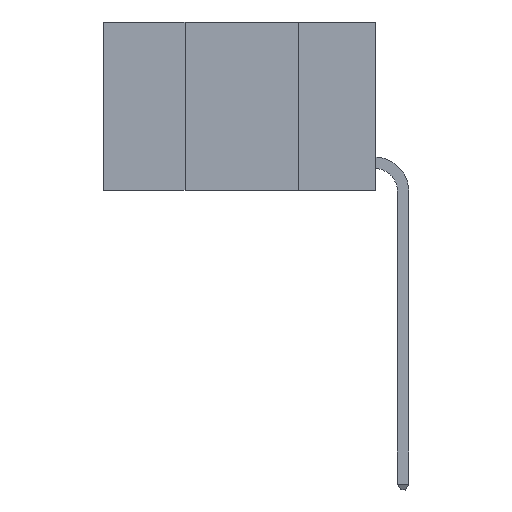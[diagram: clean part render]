
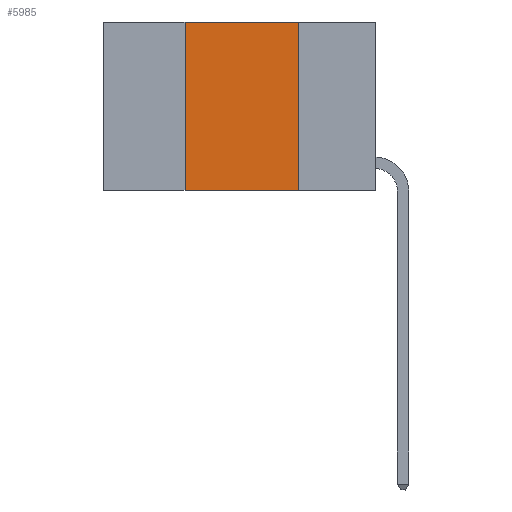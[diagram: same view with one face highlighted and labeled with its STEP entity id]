
A CAD part, left-side view. The second image highlights one B-rep face of the part: STEP entity #5985.
In plain terms, the highlighted planar face has unit normal (-1, 0, 0).
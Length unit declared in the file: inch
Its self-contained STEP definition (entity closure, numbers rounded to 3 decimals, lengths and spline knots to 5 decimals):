
#903 = EDGE_CURVE ( 'NONE', #20603, #3612, #24682, .T. ) ;
#1242 = VECTOR ( 'NONE', #6679, 39.37008 ) ;
#2431 = EDGE_LOOP ( 'NONE', ( #13528, #14172, #3925, #9391 ) ) ;
#2809 = EDGE_CURVE ( 'NONE', #20603, #3908, #10894, .T. ) ;
#2870 = VECTOR ( 'NONE', #26434, 39.37008 ) ;
#3612 = VERTEX_POINT ( 'NONE', #19601 ) ;
#3908 = VERTEX_POINT ( 'NONE', #14766 ) ;
#3925 = ORIENTED_EDGE ( 'NONE', *, *, #903, .F. ) ;
#4415 = LINE ( 'NONE', #21810, #20120 ) ;
#4591 = CARTESIAN_POINT ( 'NONE',  ( 0., 0.6, -0.37 ) ) ;
#5467 = PLANE ( 'NONE',  #12475 ) ;
#5985 = ADVANCED_FACE ( 'NONE', ( #19753 ), #5467, .F. ) ;
#6679 = DIRECTION ( 'NONE',  ( 0., -1., 0. ) ) ;
#7972 = CARTESIAN_POINT ( 'NONE',  ( 0., 0.42, -0.37 ) ) ;
#9391 = ORIENTED_EDGE ( 'NONE', *, *, #2809, .T. ) ;
#9585 = DIRECTION ( 'NONE',  ( 1., 0., 0. ) ) ;
#10894 = LINE ( 'NONE', #4591, #1242 ) ;
#12475 = AXIS2_PLACEMENT_3D ( 'NONE', #25811, #9585, #23859 ) ;
#13189 = VECTOR ( 'NONE', #19718, 39.37008 ) ;
#13528 = ORIENTED_EDGE ( 'NONE', *, *, #16050, .F. ) ;
#14172 = ORIENTED_EDGE ( 'NONE', *, *, #20093, .F. ) ;
#14766 = CARTESIAN_POINT ( 'NONE',  ( 0., 0.17, -0.37 ) ) ;
#16050 = EDGE_CURVE ( 'NONE', #23340, #3908, #24623, .T. ) ;
#16878 = CARTESIAN_POINT ( 'NONE',  ( 0., 0.17, 0. ) ) ;
#17660 = CARTESIAN_POINT ( 'NONE',  ( 0., 0.42, 0. ) ) ;
#19601 = CARTESIAN_POINT ( 'NONE',  ( 0., 0.42, 0. ) ) ;
#19718 = DIRECTION ( 'NONE',  ( 0., 0., 1. ) ) ;
#19753 = FACE_OUTER_BOUND ( 'NONE', #2431, .T. ) ;
#20093 = EDGE_CURVE ( 'NONE', #3612, #23340, #4415, .T. ) ;
#20120 = VECTOR ( 'NONE', #23864, 39.37008 ) ;
#20603 = VERTEX_POINT ( 'NONE', #7972 ) ;
#21810 = CARTESIAN_POINT ( 'NONE',  ( 0., 0.6, 0. ) ) ;
#23340 = VERTEX_POINT ( 'NONE', #16878 ) ;
#23859 = DIRECTION ( 'NONE',  ( 0., 0., -1. ) ) ;
#23864 = DIRECTION ( 'NONE',  ( 0., -1., 0. ) ) ;
#24386 = CARTESIAN_POINT ( 'NONE',  ( 0., 0.17, 0. ) ) ;
#24623 = LINE ( 'NONE', #24386, #2870 ) ;
#24682 = LINE ( 'NONE', #17660, #13189 ) ;
#25811 = CARTESIAN_POINT ( 'NONE',  ( 0., 0.6, 0. ) ) ;
#26434 = DIRECTION ( 'NONE',  ( 0., 0., -1. ) ) ;
